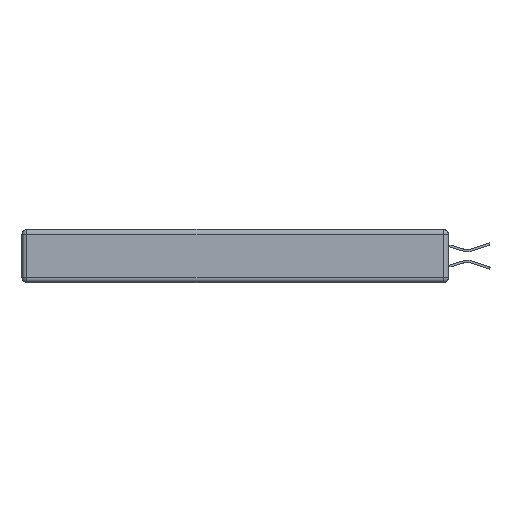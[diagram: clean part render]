
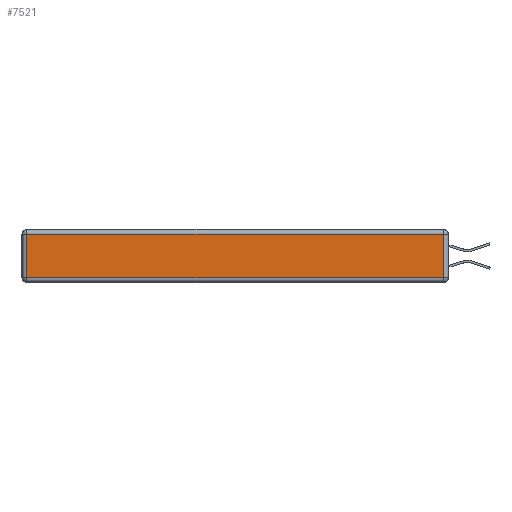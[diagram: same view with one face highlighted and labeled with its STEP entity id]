
A CAD part, left-side view. The second image highlights one B-rep face of the part: STEP entity #7521.
In plain terms, the highlighted planar face has unit normal (-1, 0, 0).
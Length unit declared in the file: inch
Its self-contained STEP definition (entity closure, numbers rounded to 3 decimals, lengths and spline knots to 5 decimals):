
#1076 = VECTOR ( 'NONE', #11563, 39.37008 ) ;
#1663 = EDGE_CURVE ( 'NONE', #19695, #5056, #22489, .T. ) ;
#2686 = LINE ( 'NONE', #19491, #1076 ) ;
#2863 = VECTOR ( 'NONE', #15824, 39.37008 ) ;
#3824 = CARTESIAN_POINT ( 'NONE',  ( 0., 0., -0.313 ) ) ;
#4886 = FACE_OUTER_BOUND ( 'NONE', #22328, .T. ) ;
#5056 = VERTEX_POINT ( 'NONE', #8630 ) ;
#5452 = DIRECTION ( 'NONE',  ( 0., 0., -1. ) ) ;
#7521 = ADVANCED_FACE ( 'NONE', ( #4886 ), #23291, .T. ) ;
#8630 = CARTESIAN_POINT ( 'NONE',  ( 0., 2.72, -0.313 ) ) ;
#8784 = ORIENTED_EDGE ( 'NONE', *, *, #18726, .T. ) ;
#9636 = DIRECTION ( 'NONE',  ( -1., 0., 0. ) ) ;
#11279 = DIRECTION ( 'NONE',  ( 0., 0., 1. ) ) ;
#11481 = CARTESIAN_POINT ( 'NONE',  ( 0., 0., -0.343 ) ) ;
#11563 = DIRECTION ( 'NONE',  ( 0., 1., 0. ) ) ;
#11612 = VECTOR ( 'NONE', #5452, 39.37008 ) ;
#12438 = VECTOR ( 'NONE', #11279, 39.37008 ) ;
#12686 = CARTESIAN_POINT ( 'NONE',  ( 0., 0.03, -0.343 ) ) ;
#13034 = LINE ( 'NONE', #12686, #12438 ) ;
#15271 = ORIENTED_EDGE ( 'NONE', *, *, #18345, .T. ) ;
#15824 = DIRECTION ( 'NONE',  ( 0., -1., 0. ) ) ;
#17145 = ORIENTED_EDGE ( 'NONE', *, *, #22958, .T. ) ;
#17635 = DIRECTION ( 'NONE',  ( 0., 0., 1. ) ) ;
#18345 = EDGE_CURVE ( 'NONE', #25326, #21697, #13034, .T. ) ;
#18444 = ORIENTED_EDGE ( 'NONE', *, *, #1663, .T. ) ;
#18726 = EDGE_CURVE ( 'NONE', #21697, #19695, #2686, .T. ) ;
#19491 = CARTESIAN_POINT ( 'NONE',  ( 0., 2.75, -0.03 ) ) ;
#19695 = VERTEX_POINT ( 'NONE', #23883 ) ;
#19758 = LINE ( 'NONE', #3824, #2863 ) ;
#20151 = AXIS2_PLACEMENT_3D ( 'NONE', #11481, #9636, #17635 ) ;
#21349 = CARTESIAN_POINT ( 'NONE',  ( 0., 0.03, -0.03 ) ) ;
#21697 = VERTEX_POINT ( 'NONE', #21349 ) ;
#22328 = EDGE_LOOP ( 'NONE', ( #17145, #15271, #8784, #18444 ) ) ;
#22489 = LINE ( 'NONE', #23207, #11612 ) ;
#22958 = EDGE_CURVE ( 'NONE', #5056, #25326, #19758, .T. ) ;
#23207 = CARTESIAN_POINT ( 'NONE',  ( 0., 2.72, -0.343 ) ) ;
#23291 = PLANE ( 'NONE',  #20151 ) ;
#23707 = CARTESIAN_POINT ( 'NONE',  ( 0., 0.03, -0.313 ) ) ;
#23883 = CARTESIAN_POINT ( 'NONE',  ( 0., 2.72, -0.03 ) ) ;
#25326 = VERTEX_POINT ( 'NONE', #23707 ) ;
